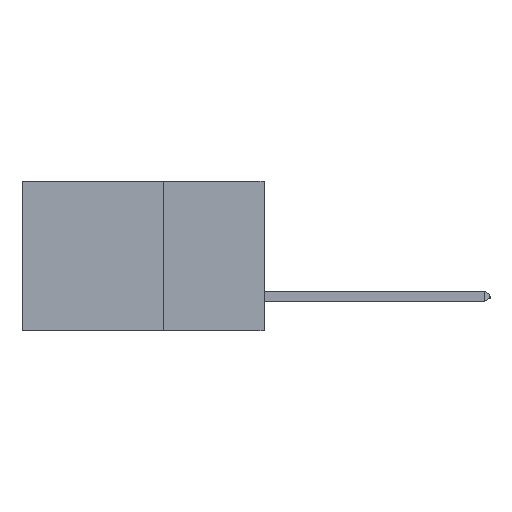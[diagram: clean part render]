
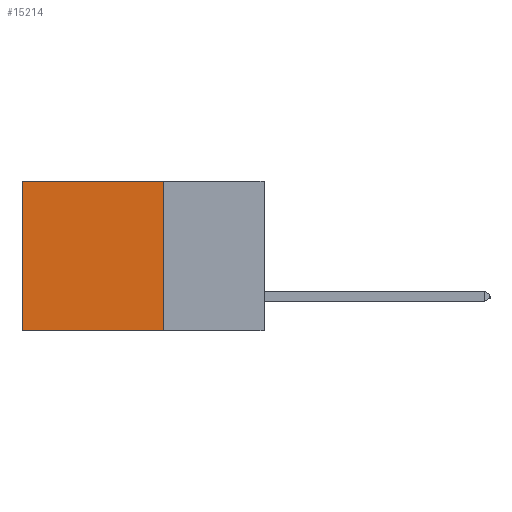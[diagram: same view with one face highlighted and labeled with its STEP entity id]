
A CAD part, left-side view. The second image highlights one B-rep face of the part: STEP entity #15214.
In plain terms, the highlighted planar face has unit normal (-1, 0, 0).
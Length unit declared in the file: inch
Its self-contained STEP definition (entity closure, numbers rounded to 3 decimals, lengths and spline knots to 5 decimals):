
#901 = EDGE_CURVE ( 'NONE', #8291, #6425, #15827, .T. ) ;
#935 = ORIENTED_EDGE ( 'NONE', *, *, #5571, .F. ) ;
#1171 = VERTEX_POINT ( 'NONE', #3230 ) ;
#1187 = EDGE_CURVE ( 'NONE', #1171, #2435, #3110, .T. ) ;
#1278 = DIRECTION ( 'NONE',  ( 0., 1., 0. ) ) ;
#2034 = CARTESIAN_POINT ( 'NONE',  ( 0.298, 0.25, 0. ) ) ;
#2435 = VERTEX_POINT ( 'NONE', #10838 ) ;
#3040 = AXIS2_PLACEMENT_3D ( 'NONE', #3549, #14117, #5175 ) ;
#3110 = LINE ( 'NONE', #3335, #18120 ) ;
#3230 = CARTESIAN_POINT ( 'NONE',  ( 0.298, 0.25, 0. ) ) ;
#3290 = VECTOR ( 'NONE', #8660, 39.37008 ) ;
#3335 = CARTESIAN_POINT ( 'NONE',  ( 0.298, 0.25, 0. ) ) ;
#3549 = CARTESIAN_POINT ( 'NONE',  ( 0.298, 0.25, 0. ) ) ;
#3877 = VECTOR ( 'NONE', #9236, 39.37008 ) ;
#3910 = CARTESIAN_POINT ( 'NONE',  ( 0.298, 0.6, -0.37 ) ) ;
#5175 = DIRECTION ( 'NONE',  ( 0., 0., -1. ) ) ;
#5571 = EDGE_CURVE ( 'NONE', #1171, #8291, #18739, .T. ) ;
#5658 = ORIENTED_EDGE ( 'NONE', *, *, #1187, .T. ) ;
#5674 = CARTESIAN_POINT ( 'NONE',  ( 0.298, 0.25, -0.37 ) ) ;
#5976 = VECTOR ( 'NONE', #8771, 39.37008 ) ;
#6425 = VERTEX_POINT ( 'NONE', #3910 ) ;
#6464 = LINE ( 'NONE', #18988, #5976 ) ;
#8291 = VERTEX_POINT ( 'NONE', #10947 ) ;
#8384 = FACE_OUTER_BOUND ( 'NONE', #14777, .T. ) ;
#8660 = DIRECTION ( 'NONE',  ( 0., 0., -1. ) ) ;
#8771 = DIRECTION ( 'NONE',  ( 0., 0., -1. ) ) ;
#9236 = DIRECTION ( 'NONE',  ( 0., 1., 0. ) ) ;
#9264 = ORIENTED_EDGE ( 'NONE', *, *, #901, .F. ) ;
#10032 = ORIENTED_EDGE ( 'NONE', *, *, #18669, .T. ) ;
#10838 = CARTESIAN_POINT ( 'NONE',  ( 0.298, 0.6, 0. ) ) ;
#10947 = CARTESIAN_POINT ( 'NONE',  ( 0.298, 0.25, -0.37 ) ) ;
#12652 = PLANE ( 'NONE',  #3040 ) ;
#14117 = DIRECTION ( 'NONE',  ( 1., 0., 0. ) ) ;
#14777 = EDGE_LOOP ( 'NONE', ( #10032, #9264, #935, #5658 ) ) ;
#15214 = ADVANCED_FACE ( 'NONE', ( #8384 ), #12652, .F. ) ;
#15827 = LINE ( 'NONE', #5674, #3877 ) ;
#18120 = VECTOR ( 'NONE', #1278, 39.37008 ) ;
#18669 = EDGE_CURVE ( 'NONE', #2435, #6425, #6464, .T. ) ;
#18739 = LINE ( 'NONE', #2034, #3290 ) ;
#18988 = CARTESIAN_POINT ( 'NONE',  ( 0.298, 0.6, 0. ) ) ;
